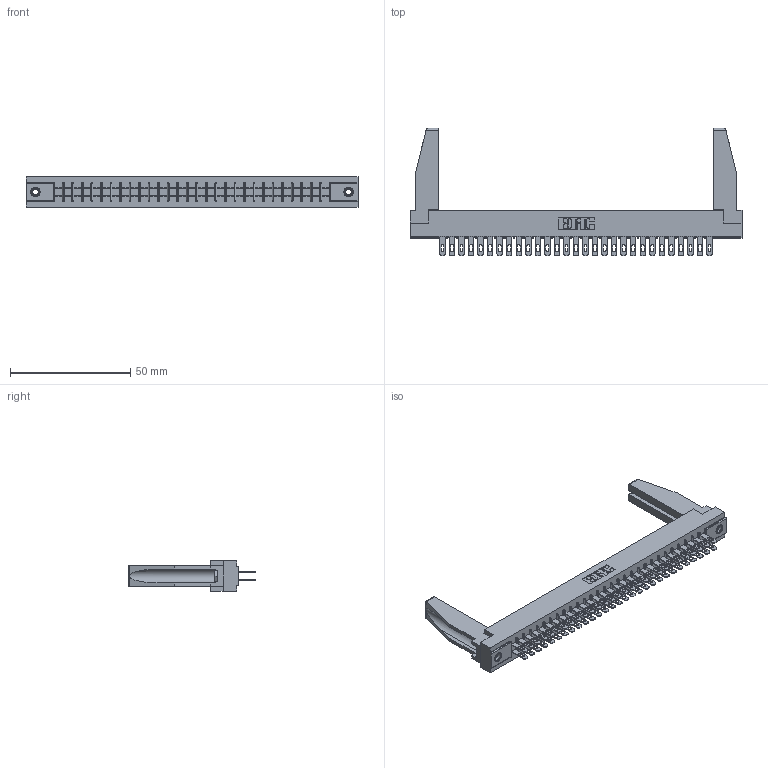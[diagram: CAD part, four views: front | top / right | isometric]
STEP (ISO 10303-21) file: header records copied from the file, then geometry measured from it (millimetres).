
FILE_DESCRIPTION (( 'STEP AP203' ), '1' );
FILE_NAME ('315-058-500-278.STEP', '2019-09-10T19:38:32', ( '' ), ( '' ), 'SwSTEP 2.0', 'SolidWorks 2016', '' );
FILE_SCHEMA (( 'CONFIG_CONTROL_DESIGN' ));
Length unit declared in the file: inch
Products named in the file (5): 307-220-078; 315-058-500-278; 345-250-001_345-250-001-102; 305 Part_.156 Dia; 305-290-001_500
Assembly tree (63 placements, depth 2):
  315-058-500-278
    305 Part_.156 Dia
    305-290-001_500  x58
    345-250-001_345-250-001-102  x2
    307-220-078  x2
Bounding box: 137.92 x 52.88 x 12.7 mm (x, y, z)
Volume: 18486.9 mm3; surface area: 23094.1 mm2
Topology: 63 solids, 63 shells, 3146 faces, 8969 edges, 5814 vertices
Faces by surface type: plane 1776, cylinder 1238, sphere 116, cone 12, torus 4
Entity records: 35443 total; most frequent: CARTESIAN_POINT 5871, ORIENTED_EDGE 5784, DIRECTION 5650, EDGE_CURVE 2892, VECTOR 2320, LINE 2320, VERTEX_POINT 1844, AXIS2_PLACEMENT_3D 1665
